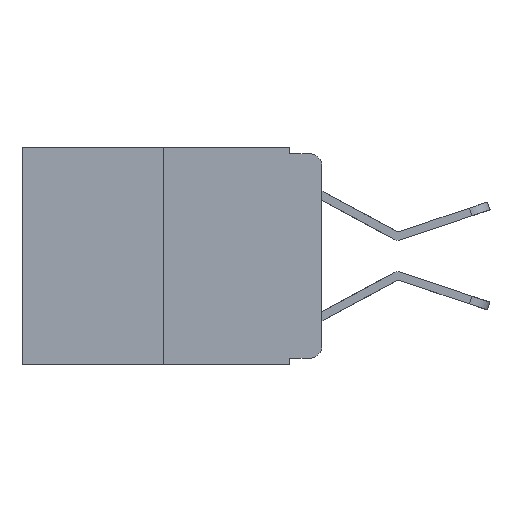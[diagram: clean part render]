
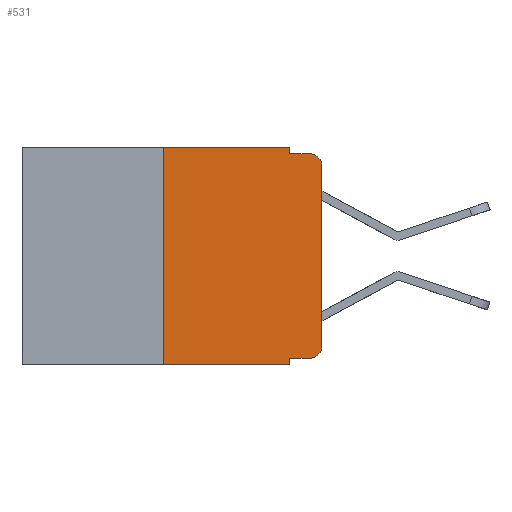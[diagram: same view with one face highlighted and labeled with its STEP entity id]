
A CAD part, left-side view. The second image highlights one B-rep face of the part: STEP entity #531.
In plain terms, the highlighted planar face has unit normal (-1, 0, 0).
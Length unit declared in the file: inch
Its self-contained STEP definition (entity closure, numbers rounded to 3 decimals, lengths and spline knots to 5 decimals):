
#531 = ADVANCED_FACE ( 'NONE', ( #16073 ), #4696, .F. ) ;
#840 = CARTESIAN_POINT ( 'NONE',  ( 0., 0.02, -0.333 ) ) ;
#1229 = ORIENTED_EDGE ( 'NONE', *, *, #6401, .T. ) ;
#1448 = CARTESIAN_POINT ( 'NONE',  ( 0., 0.051, -0.343 ) ) ;
#1721 = CARTESIAN_POINT ( 'NONE',  ( 0., 0.051, 0. ) ) ;
#2483 = VERTEX_POINT ( 'NONE', #840 ) ;
#2533 = LINE ( 'NONE', #15361, #15029 ) ;
#2620 = CIRCLE ( 'NONE', #13272, 0.02 ) ;
#2743 = AXIS2_PLACEMENT_3D ( 'NONE', #13099, #3687, #14602 ) ;
#2881 = CIRCLE ( 'NONE', #2743, 0.02 ) ;
#3261 = CARTESIAN_POINT ( 'NONE',  ( 0., 0., -0.313 ) ) ;
#3381 = DIRECTION ( 'NONE',  ( 0., 0., -1. ) ) ;
#3625 = DIRECTION ( 'NONE',  ( 0., -1., 0. ) ) ;
#3687 = DIRECTION ( 'NONE',  ( -1., 0., 0. ) ) ;
#4124 = CARTESIAN_POINT ( 'NONE',  ( 0., 0., -0.03 ) ) ;
#4536 = VERTEX_POINT ( 'NONE', #1448 ) ;
#4596 = LINE ( 'NONE', #17610, #5116 ) ;
#4696 = PLANE ( 'NONE',  #12331 ) ;
#4953 = DIRECTION ( 'NONE',  ( 0., -1., 0. ) ) ;
#5116 = VECTOR ( 'NONE', #3625, 39.37008 ) ;
#5118 = LINE ( 'NONE', #17386, #13417 ) ;
#5605 = ORIENTED_EDGE ( 'NONE', *, *, #8526, .F. ) ;
#6257 = LINE ( 'NONE', #17905, #9437 ) ;
#6401 = EDGE_CURVE ( 'NONE', #2483, #14416, #2881, .T. ) ;
#6893 = ORIENTED_EDGE ( 'NONE', *, *, #18358, .T. ) ;
#6938 = ORIENTED_EDGE ( 'NONE', *, *, #14538, .F. ) ;
#7481 = EDGE_CURVE ( 'NONE', #17935, #2483, #15575, .T. ) ;
#7534 = VERTEX_POINT ( 'NONE', #17960 ) ;
#7740 = CARTESIAN_POINT ( 'NONE',  ( 0., 0.051, -0.01 ) ) ;
#8526 = EDGE_CURVE ( 'NONE', #17935, #4536, #5118, .T. ) ;
#8542 = CARTESIAN_POINT ( 'NONE',  ( 0., 0.02, -0.01 ) ) ;
#8578 = CARTESIAN_POINT ( 'NONE',  ( 0., 0.051, -0.333 ) ) ;
#8920 = ORIENTED_EDGE ( 'NONE', *, *, #13645, .T. ) ;
#9262 = CARTESIAN_POINT ( 'NONE',  ( 0., 0.02, -0.03 ) ) ;
#9437 = VECTOR ( 'NONE', #11769, 39.37008 ) ;
#9546 = EDGE_CURVE ( 'NONE', #12705, #20093, #2533, .T. ) ;
#9630 = DIRECTION ( 'NONE',  ( 0., 0., -1. ) ) ;
#10166 = DIRECTION ( 'NONE',  ( 0., -1., 0. ) ) ;
#10557 = EDGE_CURVE ( 'NONE', #7534, #18261, #16405, .T. ) ;
#10759 = DIRECTION ( 'NONE',  ( 0., 0., -1. ) ) ;
#11240 = DIRECTION ( 'NONE',  ( 0., 0., -1. ) ) ;
#11769 = DIRECTION ( 'NONE',  ( 0., -1., 0. ) ) ;
#11821 = CARTESIAN_POINT ( 'NONE',  ( 0., 0.25, 0. ) ) ;
#12331 = AXIS2_PLACEMENT_3D ( 'NONE', #16078, #14607, #9630 ) ;
#12371 = VECTOR ( 'NONE', #11240, 39.37008 ) ;
#12570 = EDGE_LOOP ( 'NONE', ( #20045, #8920, #13201, #20267, #6938, #17367, #6893, #5605, #15998, #1229 ) ) ;
#12632 = EDGE_CURVE ( 'NONE', #18261, #17276, #6257, .T. ) ;
#12705 = VERTEX_POINT ( 'NONE', #15826 ) ;
#12761 = CARTESIAN_POINT ( 'NONE',  ( 0., 0.473, -0.343 ) ) ;
#13099 = CARTESIAN_POINT ( 'NONE',  ( 0., 0.02, -0.313 ) ) ;
#13201 = ORIENTED_EDGE ( 'NONE', *, *, #12632, .F. ) ;
#13272 = AXIS2_PLACEMENT_3D ( 'NONE', #9262, #19860, #10759 ) ;
#13417 = VECTOR ( 'NONE', #3381, 39.37008 ) ;
#13642 = VECTOR ( 'NONE', #19437, 39.37008 ) ;
#13645 = EDGE_CURVE ( 'NONE', #18113, #17276, #2620, .T. ) ;
#14416 = VERTEX_POINT ( 'NONE', #3261 ) ;
#14538 = EDGE_CURVE ( 'NONE', #20093, #7534, #4596, .T. ) ;
#14602 = DIRECTION ( 'NONE',  ( 0., 0., -1. ) ) ;
#14607 = DIRECTION ( 'NONE',  ( 1., 0., 0. ) ) ;
#14650 = EDGE_CURVE ( 'NONE', #14416, #18113, #17681, .T. ) ;
#15029 = VECTOR ( 'NONE', #19837, 39.37008 ) ;
#15269 = VECTOR ( 'NONE', #4953, 39.37008 ) ;
#15361 = CARTESIAN_POINT ( 'NONE',  ( 0., 0.25, 0. ) ) ;
#15575 = LINE ( 'NONE', #19263, #19565 ) ;
#15754 = LINE ( 'NONE', #12761, #15269 ) ;
#15826 = CARTESIAN_POINT ( 'NONE',  ( 0., 0.25, -0.343 ) ) ;
#15998 = ORIENTED_EDGE ( 'NONE', *, *, #7481, .T. ) ;
#16073 = FACE_OUTER_BOUND ( 'NONE', #12570, .T. ) ;
#16078 = CARTESIAN_POINT ( 'NONE',  ( 0., 0.473, 0. ) ) ;
#16405 = LINE ( 'NONE', #1721, #12371 ) ;
#17276 = VERTEX_POINT ( 'NONE', #8542 ) ;
#17367 = ORIENTED_EDGE ( 'NONE', *, *, #9546, .F. ) ;
#17386 = CARTESIAN_POINT ( 'NONE',  ( 0., 0.051, 0. ) ) ;
#17610 = CARTESIAN_POINT ( 'NONE',  ( 0., 0.473, 0. ) ) ;
#17681 = LINE ( 'NONE', #17936, #13642 ) ;
#17905 = CARTESIAN_POINT ( 'NONE',  ( 0., 0.051, -0.01 ) ) ;
#17935 = VERTEX_POINT ( 'NONE', #8578 ) ;
#17936 = CARTESIAN_POINT ( 'NONE',  ( 0., 0., 0. ) ) ;
#17960 = CARTESIAN_POINT ( 'NONE',  ( 0., 0.051, 0. ) ) ;
#18113 = VERTEX_POINT ( 'NONE', #4124 ) ;
#18261 = VERTEX_POINT ( 'NONE', #7740 ) ;
#18358 = EDGE_CURVE ( 'NONE', #12705, #4536, #15754, .T. ) ;
#19263 = CARTESIAN_POINT ( 'NONE',  ( 0., 0.051, -0.333 ) ) ;
#19437 = DIRECTION ( 'NONE',  ( 0., 0., 1. ) ) ;
#19565 = VECTOR ( 'NONE', #10166, 39.37008 ) ;
#19837 = DIRECTION ( 'NONE',  ( 0., 0., 1. ) ) ;
#19860 = DIRECTION ( 'NONE',  ( -1., 0., 0. ) ) ;
#20045 = ORIENTED_EDGE ( 'NONE', *, *, #14650, .T. ) ;
#20093 = VERTEX_POINT ( 'NONE', #11821 ) ;
#20267 = ORIENTED_EDGE ( 'NONE', *, *, #10557, .F. ) ;
